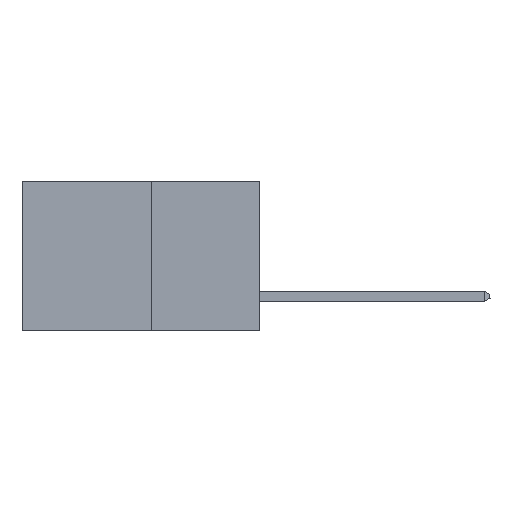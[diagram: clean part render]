
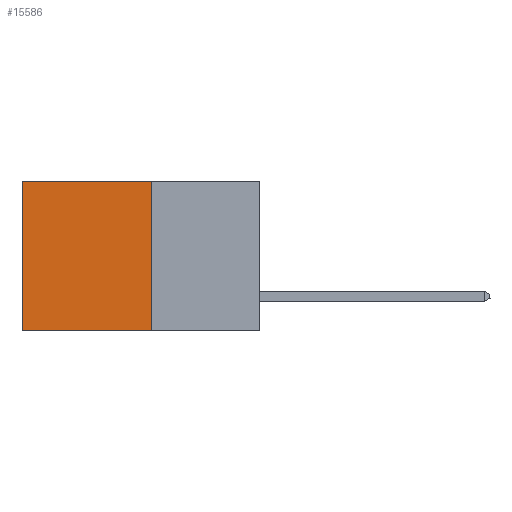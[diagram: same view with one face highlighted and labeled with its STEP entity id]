
A CAD part, left-side view. The second image highlights one B-rep face of the part: STEP entity #15586.
In plain terms, the highlighted planar face has unit normal (-1, 0, 0).
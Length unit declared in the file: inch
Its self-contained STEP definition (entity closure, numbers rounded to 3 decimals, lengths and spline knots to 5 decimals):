
#172 = EDGE_CURVE ( 'NONE', #8063, #5925, #17022, .T. ) ;
#737 = CARTESIAN_POINT ( 'NONE',  ( 0.277, 0.27, 0. ) ) ;
#788 = CARTESIAN_POINT ( 'NONE',  ( 0.277, 0.27, -0.37 ) ) ;
#868 = DIRECTION ( 'NONE',  ( 0., 1., 0. ) ) ;
#934 = EDGE_CURVE ( 'NONE', #8063, #13287, #11570, .T. ) ;
#1032 = VECTOR ( 'NONE', #12106, 39.37008 ) ;
#2165 = VECTOR ( 'NONE', #7593, 39.37008 ) ;
#2187 = VERTEX_POINT ( 'NONE', #11491 ) ;
#2664 = DIRECTION ( 'NONE',  ( 1., 0., 0. ) ) ;
#3760 = LINE ( 'NONE', #10615, #7902 ) ;
#4582 = CARTESIAN_POINT ( 'NONE',  ( 0.277, 0.27, 0. ) ) ;
#5467 = EDGE_CURVE ( 'NONE', #13287, #2187, #3760, .T. ) ;
#5801 = ORIENTED_EDGE ( 'NONE', *, *, #5467, .T. ) ;
#5925 = VERTEX_POINT ( 'NONE', #6016 ) ;
#6016 = CARTESIAN_POINT ( 'NONE',  ( 0.277, 0.27, -0.37 ) ) ;
#6030 = FACE_OUTER_BOUND ( 'NONE', #8181, .T. ) ;
#6601 = ORIENTED_EDGE ( 'NONE', *, *, #934, .T. ) ;
#7593 = DIRECTION ( 'NONE',  ( 0., 0., -1. ) ) ;
#7902 = VECTOR ( 'NONE', #10486, 39.37008 ) ;
#7932 = ORIENTED_EDGE ( 'NONE', *, *, #172, .F. ) ;
#8063 = VERTEX_POINT ( 'NONE', #737 ) ;
#8181 = EDGE_LOOP ( 'NONE', ( #5801, #8707, #7932, #6601 ) ) ;
#8707 = ORIENTED_EDGE ( 'NONE', *, *, #16539, .F. ) ;
#9177 = CARTESIAN_POINT ( 'NONE',  ( 0.277, 0.27, -0.37 ) ) ;
#10486 = DIRECTION ( 'NONE',  ( 0., 0., -1. ) ) ;
#10615 = CARTESIAN_POINT ( 'NONE',  ( 0.277, 0.59, -0.37 ) ) ;
#10839 = VECTOR ( 'NONE', #868, 39.37008 ) ;
#11229 = CARTESIAN_POINT ( 'NONE',  ( 0.277, 0.59, 0. ) ) ;
#11491 = CARTESIAN_POINT ( 'NONE',  ( 0.277, 0.59, -0.37 ) ) ;
#11570 = LINE ( 'NONE', #4582, #1032 ) ;
#12106 = DIRECTION ( 'NONE',  ( 0., 1., 0. ) ) ;
#12203 = DIRECTION ( 'NONE',  ( 0., 0., -1. ) ) ;
#13287 = VERTEX_POINT ( 'NONE', #11229 ) ;
#13974 = LINE ( 'NONE', #9177, #10839 ) ;
#14721 = AXIS2_PLACEMENT_3D ( 'NONE', #17512, #2664, #12203 ) ;
#14857 = PLANE ( 'NONE',  #14721 ) ;
#15586 = ADVANCED_FACE ( 'NONE', ( #6030 ), #14857, .F. ) ;
#16539 = EDGE_CURVE ( 'NONE', #5925, #2187, #13974, .T. ) ;
#17022 = LINE ( 'NONE', #788, #2165 ) ;
#17512 = CARTESIAN_POINT ( 'NONE',  ( 0.277, 0.27, -0.37 ) ) ;
